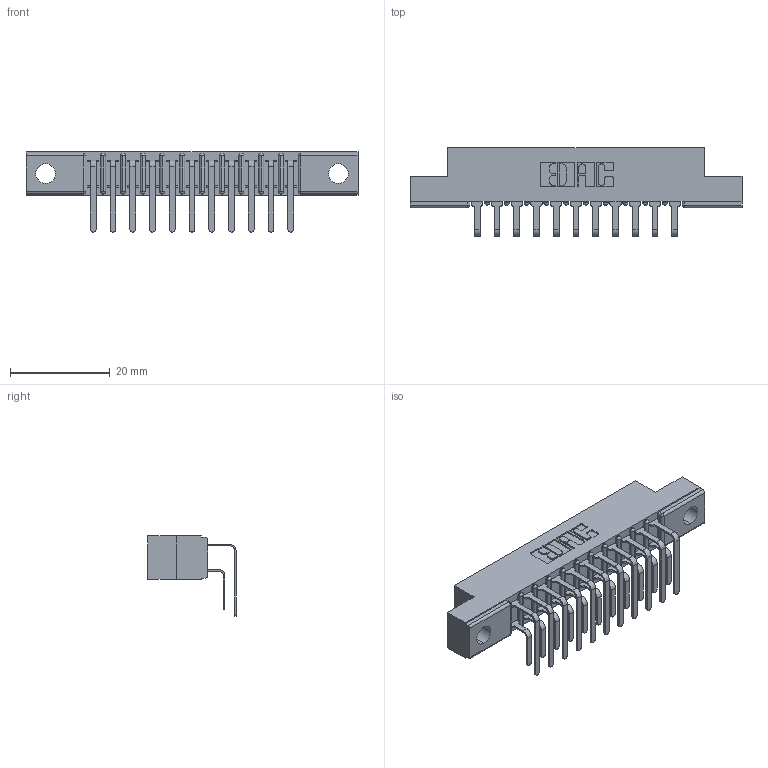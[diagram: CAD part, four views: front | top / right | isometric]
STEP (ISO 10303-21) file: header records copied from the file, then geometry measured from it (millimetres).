
FILE_DESCRIPTION (( 'STEP AP203' ), '1' );
FILE_NAME ('307-022-459-202.STEP', '2020-09-29T04:11:13', ( '' ), ( '' ), 'SwSTEP 2.0', 'SolidWorks 2020', '' );
FILE_SCHEMA (( 'CONFIG_CONTROL_DESIGN' ));
Length unit declared in the file: inch
Products named in the file (4): 307-022-459-202; 307-290-001_559 - 2 (Single); 307 Part_.128 Dia Mounting Holes; 307-290-001_558 559 - 1 (Single)
Assembly tree (23 placements, depth 2):
  307-022-459-202
    307 Part_.128 Dia Mounting Holes
    307-290-001_558 559 - 1 (Single)  x11
    307-290-001_559 - 2 (Single)  x11
Bounding box: 66.6 x 17.69 x 16.08 mm (x, y, z)
Volume: 4367.2 mm3; surface area: 7535.8 mm2
Topology: 23 solids, 23 shells, 1230 faces, 3447 edges, 2234 vertices
Faces by surface type: plane 796, cylinder 410, sphere 24
Entity records: 15053 total; most frequent: CARTESIAN_POINT 2473, ORIENTED_EDGE 2446, DIRECTION 2435, EDGE_CURVE 1223, LINE 923, VECTOR 923, VERTEX_POINT 794, AXIS2_PLACEMENT_3D 756
